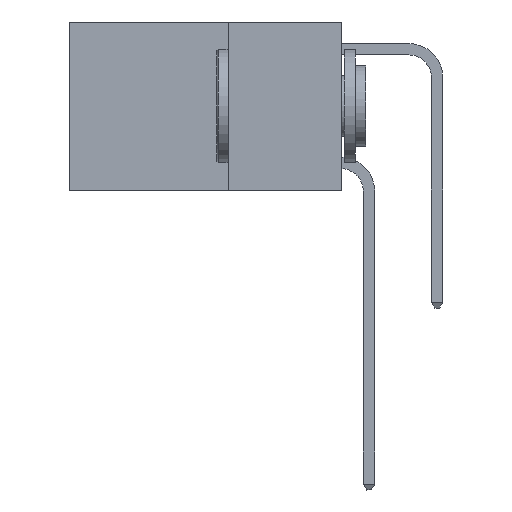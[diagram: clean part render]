
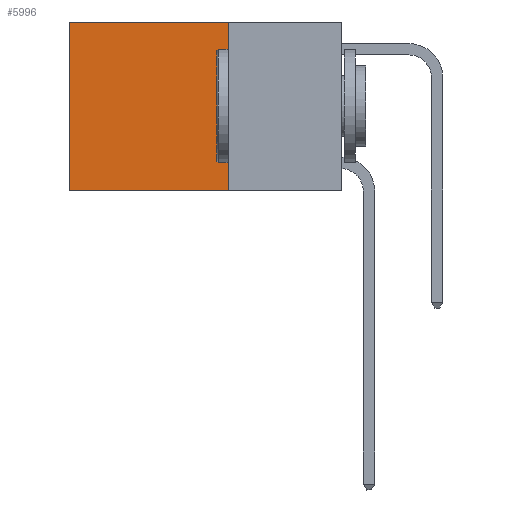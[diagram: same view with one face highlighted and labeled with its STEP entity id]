
A CAD part, left-side view. The second image highlights one B-rep face of the part: STEP entity #5996.
In plain terms, the highlighted planar face has unit normal (-1, 0, 0).
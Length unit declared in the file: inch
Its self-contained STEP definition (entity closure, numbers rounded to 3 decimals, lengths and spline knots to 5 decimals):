
#199 = DIRECTION ( 'NONE',  ( 0., 0., -1. ) ) ;
#457 = VERTEX_POINT ( 'NONE', #24695 ) ;
#840 = CARTESIAN_POINT ( 'NONE',  ( 0.2625, 0.25, 0. ) ) ;
#893 = VERTEX_POINT ( 'NONE', #3536 ) ;
#932 = VECTOR ( 'NONE', #31934, 39.37008 ) ;
#2131 = DIRECTION ( 'NONE',  ( 0., 1., 0. ) ) ;
#2710 = LINE ( 'NONE', #18273, #22146 ) ;
#3536 = CARTESIAN_POINT ( 'NONE',  ( 0.2625, 0.25, -0.37 ) ) ;
#3885 = CARTESIAN_POINT ( 'NONE',  ( 0.2625, 0.6, -0.37 ) ) ;
#4149 = VERTEX_POINT ( 'NONE', #3885 ) ;
#5162 = LINE ( 'NONE', #30715, #23706 ) ;
#5413 = DIRECTION ( 'NONE',  ( 0., 0., -1. ) ) ;
#5996 = ADVANCED_FACE ( 'NONE', ( #15407 ), #30457, .F. ) ;
#7321 = DIRECTION ( 'NONE',  ( 1., 0., 0. ) ) ;
#7862 = EDGE_CURVE ( 'NONE', #16942, #4149, #2710, .T. ) ;
#8069 = ORIENTED_EDGE ( 'NONE', *, *, #28337, .F. ) ;
#10371 = CARTESIAN_POINT ( 'NONE',  ( 0.2625, 0.25, 0. ) ) ;
#14032 = ORIENTED_EDGE ( 'NONE', *, *, #22959, .T. ) ;
#14367 = DIRECTION ( 'NONE',  ( 0., 0., -1. ) ) ;
#15407 = FACE_OUTER_BOUND ( 'NONE', #19823, .T. ) ;
#16006 = ORIENTED_EDGE ( 'NONE', *, *, #32235, .F. ) ;
#16942 = VERTEX_POINT ( 'NONE', #19622 ) ;
#18273 = CARTESIAN_POINT ( 'NONE',  ( 0.2625, 0.6, 0. ) ) ;
#19622 = CARTESIAN_POINT ( 'NONE',  ( 0.2625, 0.6, 0. ) ) ;
#19823 = EDGE_LOOP ( 'NONE', ( #20182, #8069, #16006, #14032 ) ) ;
#20182 = ORIENTED_EDGE ( 'NONE', *, *, #7862, .T. ) ;
#20382 = VECTOR ( 'NONE', #14367, 39.37008 ) ;
#20944 = LINE ( 'NONE', #24131, #932 ) ;
#21096 = AXIS2_PLACEMENT_3D ( 'NONE', #10371, #7321, #199 ) ;
#22146 = VECTOR ( 'NONE', #5413, 39.37008 ) ;
#22959 = EDGE_CURVE ( 'NONE', #457, #16942, #5162, .T. ) ;
#23706 = VECTOR ( 'NONE', #2131, 39.37008 ) ;
#24131 = CARTESIAN_POINT ( 'NONE',  ( 0.2625, 0.25, -0.37 ) ) ;
#24695 = CARTESIAN_POINT ( 'NONE',  ( 0.2625, 0.25, 0. ) ) ;
#28337 = EDGE_CURVE ( 'NONE', #893, #4149, #20944, .T. ) ;
#30457 = PLANE ( 'NONE',  #21096 ) ;
#30715 = CARTESIAN_POINT ( 'NONE',  ( 0.2625, 0.25, 0. ) ) ;
#31638 = LINE ( 'NONE', #840, #20382 ) ;
#31934 = DIRECTION ( 'NONE',  ( 0., 1., 0. ) ) ;
#32235 = EDGE_CURVE ( 'NONE', #457, #893, #31638, .T. ) ;
